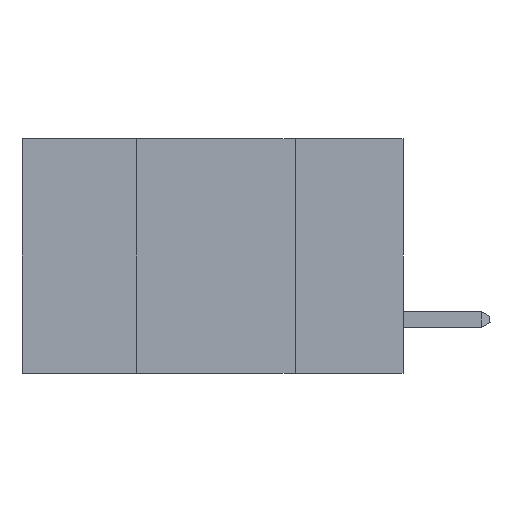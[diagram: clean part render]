
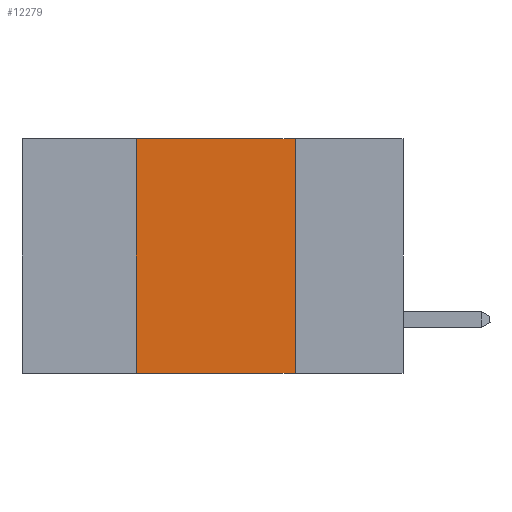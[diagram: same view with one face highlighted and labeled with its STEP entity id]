
A CAD part, left-side view. The second image highlights one B-rep face of the part: STEP entity #12279.
In plain terms, the highlighted planar face has unit normal (-1, 0, 0).
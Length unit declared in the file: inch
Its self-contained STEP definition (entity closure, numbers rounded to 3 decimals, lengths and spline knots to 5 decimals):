
#430 = DIRECTION ( 'NONE',  ( 0., -1., 0. ) ) ;
#551 = LINE ( 'NONE', #9161, #14339 ) ;
#703 = DIRECTION ( 'NONE',  ( 0., 0., -1. ) ) ;
#1620 = DIRECTION ( 'NONE',  ( 0., 0., 1. ) ) ;
#2741 = CARTESIAN_POINT ( 'NONE',  ( 0., 0.17, -0.37 ) ) ;
#2763 = VECTOR ( 'NONE', #9771, 39.37008 ) ;
#3122 = CARTESIAN_POINT ( 'NONE',  ( 0., 0.42, -0.37 ) ) ;
#3697 = PLANE ( 'NONE',  #4608 ) ;
#3745 = EDGE_CURVE ( 'NONE', #15898, #14769, #4535, .T. ) ;
#4243 = VERTEX_POINT ( 'NONE', #6781 ) ;
#4535 = LINE ( 'NONE', #5648, #8696 ) ;
#4608 = AXIS2_PLACEMENT_3D ( 'NONE', #12513, #11560, #9062 ) ;
#5003 = CARTESIAN_POINT ( 'NONE',  ( 0., 0.17, 0. ) ) ;
#5648 = CARTESIAN_POINT ( 'NONE',  ( 0., 0.17, 0. ) ) ;
#6781 = CARTESIAN_POINT ( 'NONE',  ( 0., 0.42, 0. ) ) ;
#7656 = ORIENTED_EDGE ( 'NONE', *, *, #3745, .F. ) ;
#7756 = EDGE_CURVE ( 'NONE', #14289, #4243, #551, .T. ) ;
#7988 = LINE ( 'NONE', #14399, #12174 ) ;
#8003 = EDGE_LOOP ( 'NONE', ( #7656, #14513, #10460, #8830 ) ) ;
#8076 = FACE_OUTER_BOUND ( 'NONE', #8003, .T. ) ;
#8696 = VECTOR ( 'NONE', #703, 39.37008 ) ;
#8830 = ORIENTED_EDGE ( 'NONE', *, *, #15465, .T. ) ;
#9062 = DIRECTION ( 'NONE',  ( 0., 0., -1. ) ) ;
#9161 = CARTESIAN_POINT ( 'NONE',  ( 0., 0.42, 0. ) ) ;
#9771 = DIRECTION ( 'NONE',  ( 0., -1., 0. ) ) ;
#10460 = ORIENTED_EDGE ( 'NONE', *, *, #7756, .F. ) ;
#11560 = DIRECTION ( 'NONE',  ( 1., 0., 0. ) ) ;
#12174 = VECTOR ( 'NONE', #430, 39.37008 ) ;
#12279 = ADVANCED_FACE ( 'NONE', ( #8076 ), #3697, .F. ) ;
#12513 = CARTESIAN_POINT ( 'NONE',  ( 0., 0.6, 0. ) ) ;
#13772 = LINE ( 'NONE', #16159, #2763 ) ;
#14289 = VERTEX_POINT ( 'NONE', #3122 ) ;
#14339 = VECTOR ( 'NONE', #1620, 39.37008 ) ;
#14399 = CARTESIAN_POINT ( 'NONE',  ( 0., 0.6, 0. ) ) ;
#14513 = ORIENTED_EDGE ( 'NONE', *, *, #15223, .F. ) ;
#14769 = VERTEX_POINT ( 'NONE', #2741 ) ;
#15223 = EDGE_CURVE ( 'NONE', #4243, #15898, #7988, .T. ) ;
#15465 = EDGE_CURVE ( 'NONE', #14289, #14769, #13772, .T. ) ;
#15898 = VERTEX_POINT ( 'NONE', #5003 ) ;
#16159 = CARTESIAN_POINT ( 'NONE',  ( 0., 0.6, -0.37 ) ) ;
